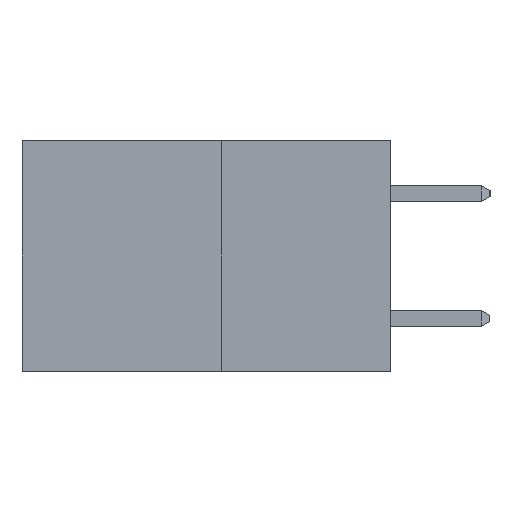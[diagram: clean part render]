
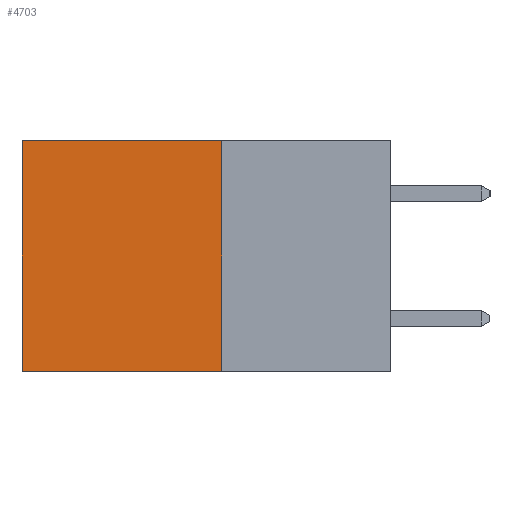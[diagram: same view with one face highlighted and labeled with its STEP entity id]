
A CAD part, left-side view. The second image highlights one B-rep face of the part: STEP entity #4703.
In plain terms, the highlighted planar face has unit normal (-1, 0, 0).
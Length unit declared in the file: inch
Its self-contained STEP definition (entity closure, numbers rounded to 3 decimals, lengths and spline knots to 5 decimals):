
#725 = CARTESIAN_POINT ( 'NONE',  ( 0.277, 0.27, -0.37 ) ) ;
#898 = CARTESIAN_POINT ( 'NONE',  ( 0.277, 0.59, -0.37 ) ) ;
#1262 = VECTOR ( 'NONE', #5829, 39.37008 ) ;
#1789 = CARTESIAN_POINT ( 'NONE',  ( 0.277, 0.27, -0.37 ) ) ;
#2587 = CARTESIAN_POINT ( 'NONE',  ( 0.277, 0.27, 0. ) ) ;
#2699 = DIRECTION ( 'NONE',  ( 0., 0., -1. ) ) ;
#2838 = VERTEX_POINT ( 'NONE', #6899 ) ;
#3032 = EDGE_CURVE ( 'NONE', #3258, #2838, #11822, .T. ) ;
#3171 = VECTOR ( 'NONE', #11845, 39.37008 ) ;
#3258 = VERTEX_POINT ( 'NONE', #6372 ) ;
#3269 = LINE ( 'NONE', #9668, #13355 ) ;
#3782 = CARTESIAN_POINT ( 'NONE',  ( 0.277, 0.27, 0. ) ) ;
#3808 = VERTEX_POINT ( 'NONE', #6394 ) ;
#4450 = ORIENTED_EDGE ( 'NONE', *, *, #5249, .F. ) ;
#4703 = ADVANCED_FACE ( 'NONE', ( #4960 ), #7569, .F. ) ;
#4960 = FACE_OUTER_BOUND ( 'NONE', #10730, .T. ) ;
#5017 = LINE ( 'NONE', #1789, #12037 ) ;
#5249 = EDGE_CURVE ( 'NONE', #7312, #3808, #3269, .T. ) ;
#5363 = AXIS2_PLACEMENT_3D ( 'NONE', #725, #6319, #2699 ) ;
#5829 = DIRECTION ( 'NONE',  ( 0., 0., -1. ) ) ;
#6319 = DIRECTION ( 'NONE',  ( 1., 0., 0. ) ) ;
#6372 = CARTESIAN_POINT ( 'NONE',  ( 0.277, 0.59, 0. ) ) ;
#6394 = CARTESIAN_POINT ( 'NONE',  ( 0.277, 0.27, -0.37 ) ) ;
#6899 = CARTESIAN_POINT ( 'NONE',  ( 0.277, 0.59, -0.37 ) ) ;
#7312 = VERTEX_POINT ( 'NONE', #3782 ) ;
#7569 = PLANE ( 'NONE',  #5363 ) ;
#8861 = DIRECTION ( 'NONE',  ( 0., 0., -1. ) ) ;
#9668 = CARTESIAN_POINT ( 'NONE',  ( 0.277, 0.27, -0.37 ) ) ;
#10730 = EDGE_LOOP ( 'NONE', ( #13233, #16071, #4450, #10857 ) ) ;
#10857 = ORIENTED_EDGE ( 'NONE', *, *, #11384, .T. ) ;
#11384 = EDGE_CURVE ( 'NONE', #7312, #3258, #16150, .T. ) ;
#11822 = LINE ( 'NONE', #898, #1262 ) ;
#11845 = DIRECTION ( 'NONE',  ( 0., 1., 0. ) ) ;
#12037 = VECTOR ( 'NONE', #14827, 39.37008 ) ;
#13058 = EDGE_CURVE ( 'NONE', #3808, #2838, #5017, .T. ) ;
#13233 = ORIENTED_EDGE ( 'NONE', *, *, #3032, .T. ) ;
#13355 = VECTOR ( 'NONE', #8861, 39.37008 ) ;
#14827 = DIRECTION ( 'NONE',  ( 0., 1., 0. ) ) ;
#16071 = ORIENTED_EDGE ( 'NONE', *, *, #13058, .F. ) ;
#16150 = LINE ( 'NONE', #2587, #3171 ) ;
